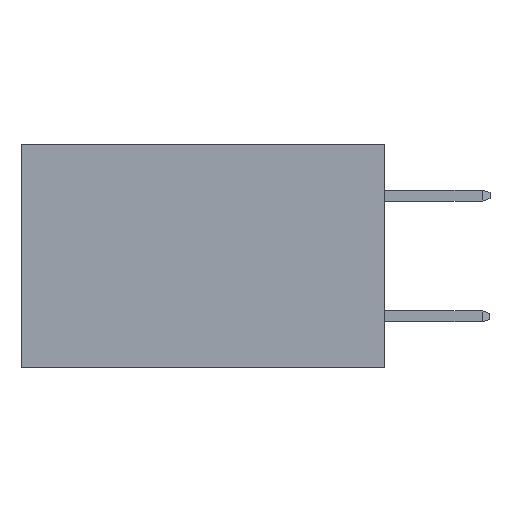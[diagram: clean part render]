
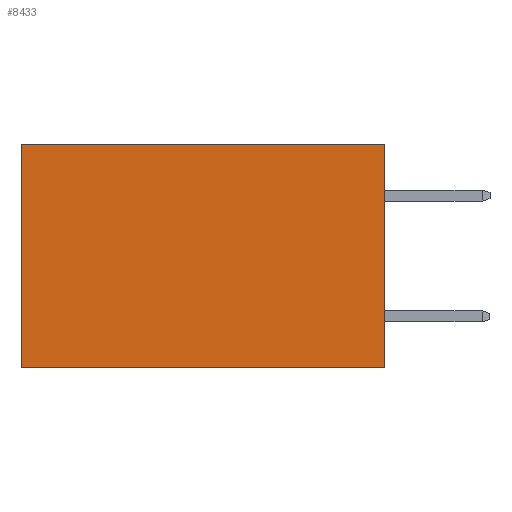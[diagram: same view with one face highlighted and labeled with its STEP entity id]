
A CAD part, left-side view. The second image highlights one B-rep face of the part: STEP entity #8433.
In plain terms, the highlighted planar face has unit normal (-1, 0, 0).
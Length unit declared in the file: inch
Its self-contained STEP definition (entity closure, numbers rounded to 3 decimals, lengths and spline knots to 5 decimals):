
#553 = ORIENTED_EDGE ( 'NONE', *, *, #6779, .F. ) ;
#1160 = CARTESIAN_POINT ( 'NONE',  ( 0.298, 0.6, 0. ) ) ;
#2094 = VECTOR ( 'NONE', #7352, 39.37008 ) ;
#2639 = DIRECTION ( 'NONE',  ( 0., 0., -1. ) ) ;
#3274 = FACE_OUTER_BOUND ( 'NONE', #9545, .T. ) ;
#3381 = VERTEX_POINT ( 'NONE', #1160 ) ;
#3523 = DIRECTION ( 'NONE',  ( 0., 1., 0. ) ) ;
#4387 = DIRECTION ( 'NONE',  ( 1., 0., 0. ) ) ;
#6659 = ORIENTED_EDGE ( 'NONE', *, *, #19335, .T. ) ;
#6779 = EDGE_CURVE ( 'NONE', #19255, #27351, #10591, .T. ) ;
#7352 = DIRECTION ( 'NONE',  ( 0., 1., 0. ) ) ;
#8433 = ADVANCED_FACE ( 'NONE', ( #3274 ), #27893, .F. ) ;
#8674 = ORIENTED_EDGE ( 'NONE', *, *, #22806, .F. ) ;
#9327 = CARTESIAN_POINT ( 'NONE',  ( 0.298, 0.6, 0. ) ) ;
#9545 = EDGE_LOOP ( 'NONE', ( #13485, #553, #8674, #6659 ) ) ;
#9601 = VECTOR ( 'NONE', #2639, 39.37008 ) ;
#9868 = VERTEX_POINT ( 'NONE', #24471 ) ;
#10591 = LINE ( 'NONE', #28219, #21634 ) ;
#11566 = VECTOR ( 'NONE', #16670, 39.37008 ) ;
#13485 = ORIENTED_EDGE ( 'NONE', *, *, #15126, .T. ) ;
#15126 = EDGE_CURVE ( 'NONE', #3381, #27351, #21329, .T. ) ;
#15322 = CARTESIAN_POINT ( 'NONE',  ( 0.298, 0.6, -0.37 ) ) ;
#16107 = CARTESIAN_POINT ( 'NONE',  ( 0.298, 0., 0. ) ) ;
#16670 = DIRECTION ( 'NONE',  ( 0., 0., -1. ) ) ;
#17438 = LINE ( 'NONE', #27559, #11566 ) ;
#19255 = VERTEX_POINT ( 'NONE', #24661 ) ;
#19335 = EDGE_CURVE ( 'NONE', #9868, #3381, #25516, .T. ) ;
#21329 = LINE ( 'NONE', #9327, #9601 ) ;
#21634 = VECTOR ( 'NONE', #3523, 39.37008 ) ;
#22806 = EDGE_CURVE ( 'NONE', #9868, #19255, #17438, .T. ) ;
#24471 = CARTESIAN_POINT ( 'NONE',  ( 0.298, 0., 0. ) ) ;
#24661 = CARTESIAN_POINT ( 'NONE',  ( 0.298, 0., -0.37 ) ) ;
#25481 = DIRECTION ( 'NONE',  ( 0., 0., -1. ) ) ;
#25516 = LINE ( 'NONE', #16107, #2094 ) ;
#27351 = VERTEX_POINT ( 'NONE', #15322 ) ;
#27535 = AXIS2_PLACEMENT_3D ( 'NONE', #27836, #4387, #25481 ) ;
#27559 = CARTESIAN_POINT ( 'NONE',  ( 0.298, 0., 0. ) ) ;
#27836 = CARTESIAN_POINT ( 'NONE',  ( 0.298, 0., 0. ) ) ;
#27893 = PLANE ( 'NONE',  #27535 ) ;
#28219 = CARTESIAN_POINT ( 'NONE',  ( 0.298, 0., -0.37 ) ) ;
